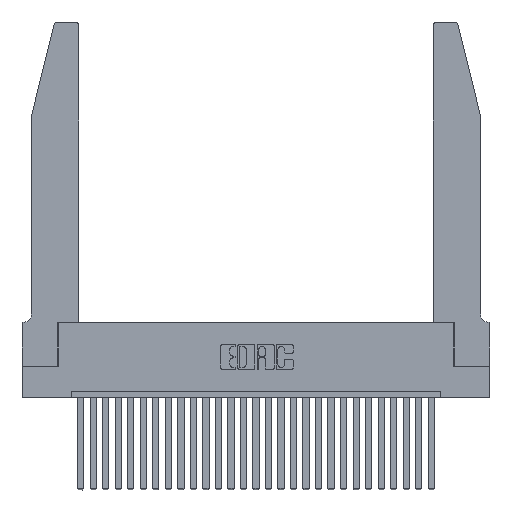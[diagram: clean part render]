
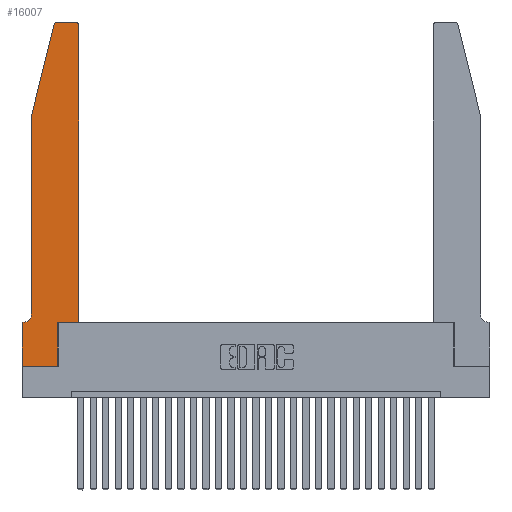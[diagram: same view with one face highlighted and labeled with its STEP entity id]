
A CAD part, top view. The second image highlights one B-rep face of the part: STEP entity #16007.
In plain terms, the highlighted planar face has unit normal (0, 0, 1).
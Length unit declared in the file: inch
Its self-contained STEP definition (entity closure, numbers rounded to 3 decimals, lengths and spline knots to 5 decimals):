
#49 = ORIENTED_EDGE ( 'NONE', *, *, #7033, .T. ) ;
#524 = LINE ( 'NONE', #1452, #25035 ) ;
#528 = CARTESIAN_POINT ( 'NONE',  ( 0.0055, 0.35, 0.37 ) ) ;
#796 = VECTOR ( 'NONE', #9227, 39.37008 ) ;
#947 = CARTESIAN_POINT ( 'NONE',  ( 0.25487, 2.72718, 0.37 ) ) ;
#1306 = CIRCLE ( 'NONE', #28061, 0.03 ) ;
#1452 = CARTESIAN_POINT ( 'NONE',  ( 0.4505, 0.35, 0.37 ) ) ;
#2430 = EDGE_CURVE ( 'NONE', #13144, #27352, #24068, .T. ) ;
#2596 = CARTESIAN_POINT ( 'NONE',  ( 0., 0., 0.37 ) ) ;
#2747 = VERTEX_POINT ( 'NONE', #528 ) ;
#3176 = LINE ( 'NONE', #11505, #796 ) ;
#3591 = DIRECTION ( 'NONE',  ( 0., 0., 1. ) ) ;
#4010 = VECTOR ( 'NONE', #26422, 39.37008 ) ;
#4250 = ORIENTED_EDGE ( 'NONE', *, *, #4914, .T. ) ;
#4273 = LINE ( 'NONE', #2596, #5931 ) ;
#4524 = CARTESIAN_POINT ( 'NONE',  ( 0.0755, 2., 0.37 ) ) ;
#4697 = VECTOR ( 'NONE', #15720, 39.37008 ) ;
#4827 = CARTESIAN_POINT ( 'NONE',  ( 0.0055, 0.42, 0.37 ) ) ;
#4914 = EDGE_CURVE ( 'NONE', #11335, #9455, #26955, .T. ) ;
#5209 = ORIENTED_EDGE ( 'NONE', *, *, #26982, .T. ) ;
#5527 = DIRECTION ( 'NONE',  ( -1., 0., 0. ) ) ;
#5624 = LINE ( 'NONE', #16403, #16813 ) ;
#5661 = CARTESIAN_POINT ( 'NONE',  ( 0., 0.35, 0.37 ) ) ;
#5846 = PLANE ( 'NONE',  #27100 ) ;
#5931 = VECTOR ( 'NONE', #23981, 39.37008 ) ;
#5968 = CARTESIAN_POINT ( 'NONE',  ( 0., 0.35, 0.37 ) ) ;
#6278 = ORIENTED_EDGE ( 'NONE', *, *, #24228, .T. ) ;
#6620 = CARTESIAN_POINT ( 'NONE',  ( 0.284, 2.75, 0.37 ) ) ;
#7033 = EDGE_CURVE ( 'NONE', #2747, #13824, #5624, .T. ) ;
#7042 = CARTESIAN_POINT ( 'NONE',  ( 0.2865, 0.35, 0.37 ) ) ;
#8431 = DIRECTION ( 'NONE',  ( -0.239, -0.971, 0. ) ) ;
#8871 = DIRECTION ( 'NONE',  ( 0., -1., 0. ) ) ;
#9048 = CARTESIAN_POINT ( 'NONE',  ( 0., 0., 0.37 ) ) ;
#9211 = ORIENTED_EDGE ( 'NONE', *, *, #11117, .T. ) ;
#9227 = DIRECTION ( 'NONE',  ( -1., 0., 0. ) ) ;
#9367 = ORIENTED_EDGE ( 'NONE', *, *, #19285, .T. ) ;
#9455 = VERTEX_POINT ( 'NONE', #21277 ) ;
#9486 = VERTEX_POINT ( 'NONE', #16848 ) ;
#9591 = VECTOR ( 'NONE', #8431, 39.37008 ) ;
#9615 = DIRECTION ( 'NONE',  ( 1., 0., 0. ) ) ;
#9667 = ORIENTED_EDGE ( 'NONE', *, *, #14030, .T. ) ;
#9858 = FACE_OUTER_BOUND ( 'NONE', #12032, .T. ) ;
#10084 = CARTESIAN_POINT ( 'NONE',  ( 0.4505, 2.72, 0.37 ) ) ;
#10121 = DIRECTION ( 'NONE',  ( 1., 0., 0. ) ) ;
#11117 = EDGE_CURVE ( 'NONE', #9486, #18165, #12795, .T. ) ;
#11335 = VERTEX_POINT ( 'NONE', #947 ) ;
#11370 = CARTESIAN_POINT ( 'NONE',  ( 0.4205, 2.75, 0.37 ) ) ;
#11451 = VECTOR ( 'NONE', #15853, 39.37008 ) ;
#11453 = DIRECTION ( 'NONE',  ( 0., 0., -1. ) ) ;
#11505 = CARTESIAN_POINT ( 'NONE',  ( 0.2605, 2.75, 0.37 ) ) ;
#11690 = LINE ( 'NONE', #4524, #23641 ) ;
#11895 = ORIENTED_EDGE ( 'NONE', *, *, #25671, .T. ) ;
#12032 = EDGE_LOOP ( 'NONE', ( #9667, #9367, #4250, #5209, #6278, #49, #11895, #12563, #9211, #24049, #17584, #22087 ) ) ;
#12563 = ORIENTED_EDGE ( 'NONE', *, *, #21265, .T. ) ;
#12707 = CARTESIAN_POINT ( 'NONE',  ( 0.4205, 2.72, 0.37 ) ) ;
#12795 = LINE ( 'NONE', #7042, #4697 ) ;
#12802 = AXIS2_PLACEMENT_3D ( 'NONE', #4827, #11453, #26697 ) ;
#13069 = CIRCLE ( 'NONE', #24202, 0.03 ) ;
#13144 = VERTEX_POINT ( 'NONE', #21073 ) ;
#13824 = VERTEX_POINT ( 'NONE', #5968 ) ;
#14030 = EDGE_CURVE ( 'NONE', #17551, #24182, #3176, .T. ) ;
#14090 = LINE ( 'NONE', #17725, #4010 ) ;
#15720 = DIRECTION ( 'NONE',  ( 0., 1., 0. ) ) ;
#15853 = DIRECTION ( 'NONE',  ( 0., 1., 0. ) ) ;
#15880 = CARTESIAN_POINT ( 'NONE',  ( 0.0755, 0.42, 0.37 ) ) ;
#16007 = ADVANCED_FACE ( 'NONE', ( #9858 ), #5846, .T. ) ;
#16403 = CARTESIAN_POINT ( 'NONE',  ( 0.0755, 0.35, 0.37 ) ) ;
#16813 = VECTOR ( 'NONE', #5527, 39.37008 ) ;
#16848 = CARTESIAN_POINT ( 'NONE',  ( 0.2865, 0., 0.37 ) ) ;
#17551 = VERTEX_POINT ( 'NONE', #11370 ) ;
#17584 = ORIENTED_EDGE ( 'NONE', *, *, #2430, .T. ) ;
#17725 = CARTESIAN_POINT ( 'NONE',  ( 0., 0., 0.37 ) ) ;
#18165 = VERTEX_POINT ( 'NONE', #18383 ) ;
#18258 = CARTESIAN_POINT ( 'NONE',  ( 0.284, 2.72, 0.37 ) ) ;
#18383 = CARTESIAN_POINT ( 'NONE',  ( 0.2865, 0.35, 0.37 ) ) ;
#19285 = EDGE_CURVE ( 'NONE', #24182, #11335, #1306, .T. ) ;
#20737 = CIRCLE ( 'NONE', #12802, 0.07 ) ;
#21073 = CARTESIAN_POINT ( 'NONE',  ( 0.4505, 0.35, 0.37 ) ) ;
#21265 = EDGE_CURVE ( 'NONE', #27022, #9486, #4273, .T. ) ;
#21277 = CARTESIAN_POINT ( 'NONE',  ( 0.0755, 2., 0.37 ) ) ;
#22087 = ORIENTED_EDGE ( 'NONE', *, *, #26059, .T. ) ;
#22212 = CARTESIAN_POINT ( 'NONE',  ( 0.4505, 0.35, 0.37 ) ) ;
#22664 = DIRECTION ( 'NONE',  ( 0., 0., 1. ) ) ;
#23641 = VECTOR ( 'NONE', #8871, 39.37008 ) ;
#23898 = DIRECTION ( 'NONE',  ( 0., 0., 1. ) ) ;
#23981 = DIRECTION ( 'NONE',  ( 1., 0., 0. ) ) ;
#24049 = ORIENTED_EDGE ( 'NONE', *, *, #26652, .T. ) ;
#24068 = LINE ( 'NONE', #22212, #11451 ) ;
#24182 = VERTEX_POINT ( 'NONE', #6620 ) ;
#24202 = AXIS2_PLACEMENT_3D ( 'NONE', #12707, #23898, #25993 ) ;
#24228 = EDGE_CURVE ( 'NONE', #24306, #2747, #20737, .T. ) ;
#24306 = VERTEX_POINT ( 'NONE', #15880 ) ;
#25035 = VECTOR ( 'NONE', #10121, 39.37008 ) ;
#25263 = DIRECTION ( 'NONE',  ( 1., 0., 0. ) ) ;
#25671 = EDGE_CURVE ( 'NONE', #13824, #27022, #14090, .T. ) ;
#25993 = DIRECTION ( 'NONE',  ( 1., 0., 0. ) ) ;
#26059 = EDGE_CURVE ( 'NONE', #27352, #17551, #13069, .T. ) ;
#26422 = DIRECTION ( 'NONE',  ( 0., -1., 0. ) ) ;
#26652 = EDGE_CURVE ( 'NONE', #18165, #13144, #524, .T. ) ;
#26697 = DIRECTION ( 'NONE',  ( -1., 0., 0. ) ) ;
#26955 = LINE ( 'NONE', #27648, #9591 ) ;
#26982 = EDGE_CURVE ( 'NONE', #9455, #24306, #11690, .T. ) ;
#27022 = VERTEX_POINT ( 'NONE', #9048 ) ;
#27100 = AXIS2_PLACEMENT_3D ( 'NONE', #5661, #3591, #25263 ) ;
#27352 = VERTEX_POINT ( 'NONE', #10084 ) ;
#27648 = CARTESIAN_POINT ( 'NONE',  ( 0.0755, 2., 0.37 ) ) ;
#28061 = AXIS2_PLACEMENT_3D ( 'NONE', #18258, #22664, #9615 ) ;
